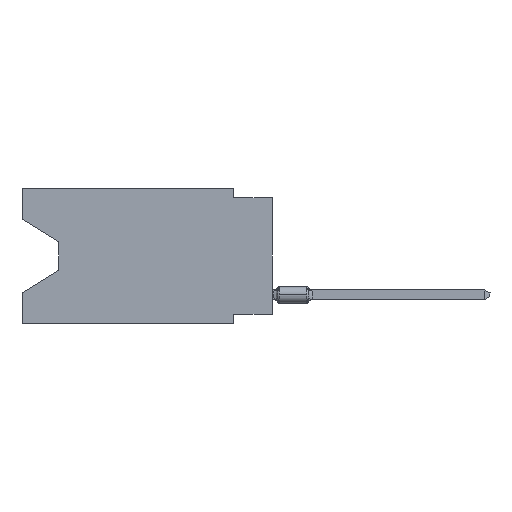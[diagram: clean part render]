
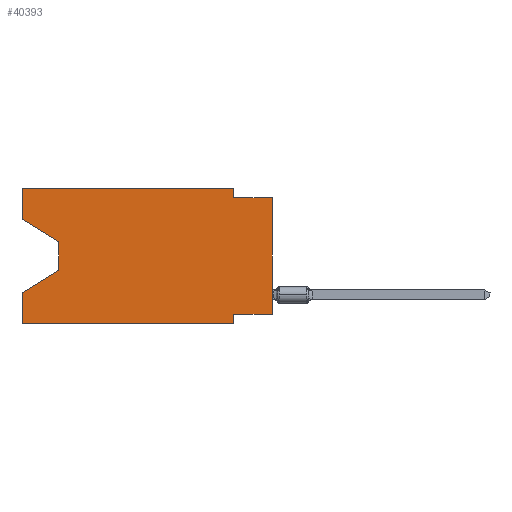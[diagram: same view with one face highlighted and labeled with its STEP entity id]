
A CAD part, left-side view. The second image highlights one B-rep face of the part: STEP entity #40393.
In plain terms, the highlighted planar face has unit normal (-1, 0, 0).
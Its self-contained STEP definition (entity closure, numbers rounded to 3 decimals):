
#534 = CARTESIAN_POINT ( 'NONE',  ( 0., 16.383, 0. ) ) ;
#1116 = CARTESIAN_POINT ( 'NONE',  ( 0., 16.383, 0. ) ) ;
#1159 = LINE ( 'NONE', #534, #43737 ) ;
#1379 = LINE ( 'NONE', #24258, #45054 ) ;
#1536 = DIRECTION ( 'NONE',  ( 0., 0., -1. ) ) ;
#2438 = EDGE_LOOP ( 'NONE', ( #58298, #54581, #25618, #20594, #7840, #58478, #11029, #13163, #11978, #22120, #38118, #57134 ) ) ;
#2689 = EDGE_CURVE ( 'NONE', #57153, #38139, #52926, .T. ) ;
#3599 = EDGE_CURVE ( 'NONE', #52192, #25789, #53669, .T. ) ;
#4442 = VECTOR ( 'NONE', #15728, 1000. ) ;
#5353 = DIRECTION ( 'NONE',  ( 0., 0., -1. ) ) ;
#6233 = FACE_OUTER_BOUND ( 'NONE', #2438, .T. ) ;
#7737 = EDGE_CURVE ( 'NONE', #38989, #37722, #52046, .T. ) ;
#7840 = ORIENTED_EDGE ( 'NONE', *, *, #38805, .T. ) ;
#7845 = CARTESIAN_POINT ( 'NONE',  ( 0., 13.97, -5.385 ) ) ;
#9365 = DIRECTION ( 'NONE',  ( 0., 0., 1. ) ) ;
#10062 = VERTEX_POINT ( 'NONE', #35258 ) ;
#10211 = CARTESIAN_POINT ( 'NONE',  ( 0., 16.383, 0. ) ) ;
#11029 = ORIENTED_EDGE ( 'NONE', *, *, #59917, .F. ) ;
#11051 = EDGE_CURVE ( 'NONE', #14133, #39056, #57338, .T. ) ;
#11978 = ORIENTED_EDGE ( 'NONE', *, *, #13653, .F. ) ;
#12089 = LINE ( 'NONE', #25820, #41133 ) ;
#12208 = CARTESIAN_POINT ( 'NONE',  ( 0., 16.383, -8.89 ) ) ;
#13156 = EDGE_CURVE ( 'NONE', #53012, #34912, #12089, .T. ) ;
#13163 = ORIENTED_EDGE ( 'NONE', *, *, #3599, .T. ) ;
#13304 = EDGE_CURVE ( 'NONE', #10062, #37722, #45962, .T. ) ;
#13653 = EDGE_CURVE ( 'NONE', #48090, #25789, #21405, .T. ) ;
#13807 = EDGE_CURVE ( 'NONE', #38139, #48090, #1379, .T. ) ;
#14133 = VERTEX_POINT ( 'NONE', #50762 ) ;
#15728 = DIRECTION ( 'NONE',  ( 0., -1., 0. ) ) ;
#16713 = VECTOR ( 'NONE', #56266, 1000. ) ;
#17088 = LINE ( 'NONE', #12208, #52303 ) ;
#19341 = CARTESIAN_POINT ( 'NONE',  ( 0., 2.54, -0.635 ) ) ;
#19373 = CARTESIAN_POINT ( 'NONE',  ( 0., 16.383, -2.038 ) ) ;
#20360 = DIRECTION ( 'NONE',  ( 0., -0.855, -0.519 ) ) ;
#20594 = ORIENTED_EDGE ( 'NONE', *, *, #7737, .F. ) ;
#21405 = LINE ( 'NONE', #31171, #56774 ) ;
#21551 = DIRECTION ( 'NONE',  ( 0., 0.855, -0.519 ) ) ;
#22120 = ORIENTED_EDGE ( 'NONE', *, *, #13807, .F. ) ;
#23295 = EDGE_CURVE ( 'NONE', #53012, #57153, #1159, .T. ) ;
#24258 = CARTESIAN_POINT ( 'NONE',  ( 0., 2.54, 0. ) ) ;
#24838 = PLANE ( 'NONE',  #38788 ) ;
#24875 = DIRECTION ( 'NONE',  ( 0., -1., 0. ) ) ;
#25618 = ORIENTED_EDGE ( 'NONE', *, *, #13304, .T. ) ;
#25625 = DIRECTION ( 'NONE',  ( 0., 0., 1. ) ) ;
#25789 = VERTEX_POINT ( 'NONE', #59652 ) ;
#25820 = CARTESIAN_POINT ( 'NONE',  ( 0., 16.383, -2.038 ) ) ;
#26841 = CARTESIAN_POINT ( 'NONE',  ( 0., 16.383, -6.852 ) ) ;
#26843 = VECTOR ( 'NONE', #51600, 1000. ) ;
#27988 = DIRECTION ( 'NONE',  ( 0., 0., 1. ) ) ;
#28391 = CARTESIAN_POINT ( 'NONE',  ( 0., 0., -8.255 ) ) ;
#31171 = CARTESIAN_POINT ( 'NONE',  ( 0., 0., -0.635 ) ) ;
#34187 = EDGE_CURVE ( 'NONE', #34912, #10062, #51899, .T. ) ;
#34273 = DIRECTION ( 'NONE',  ( 1., 0., 0. ) ) ;
#34309 = CARTESIAN_POINT ( 'NONE',  ( 0., 16.383, 0. ) ) ;
#34912 = VERTEX_POINT ( 'NONE', #37631 ) ;
#35258 = CARTESIAN_POINT ( 'NONE',  ( 0., 13.97, -5.385 ) ) ;
#37631 = CARTESIAN_POINT ( 'NONE',  ( 0., 13.97, -3.505 ) ) ;
#37722 = VERTEX_POINT ( 'NONE', #26841 ) ;
#37968 = VECTOR ( 'NONE', #9365, 1000. ) ;
#38118 = ORIENTED_EDGE ( 'NONE', *, *, #2689, .F. ) ;
#38139 = VERTEX_POINT ( 'NONE', #45071 ) ;
#38788 = AXIS2_PLACEMENT_3D ( 'NONE', #47718, #34273, #48309 ) ;
#38805 = EDGE_CURVE ( 'NONE', #38989, #39056, #17088, .T. ) ;
#38989 = VERTEX_POINT ( 'NONE', #40880 ) ;
#39056 = VERTEX_POINT ( 'NONE', #56095 ) ;
#39057 = CARTESIAN_POINT ( 'NONE',  ( 0., 0., 0. ) ) ;
#40393 = ADVANCED_FACE ( 'NONE', ( #6233 ), #24838, .F. ) ;
#40880 = CARTESIAN_POINT ( 'NONE',  ( 0., 16.383, -8.89 ) ) ;
#41133 = VECTOR ( 'NONE', #20360, 1000. ) ;
#42539 = CARTESIAN_POINT ( 'NONE',  ( 0., 0., -8.255 ) ) ;
#43737 = VECTOR ( 'NONE', #27988, 1000. ) ;
#45054 = VECTOR ( 'NONE', #5353, 1000. ) ;
#45071 = CARTESIAN_POINT ( 'NONE',  ( 0., 2.54, 0. ) ) ;
#45962 = LINE ( 'NONE', #7845, #47948 ) ;
#47718 = CARTESIAN_POINT ( 'NONE',  ( 0., 16.383, 0. ) ) ;
#47948 = VECTOR ( 'NONE', #21551, 1000. ) ;
#48090 = VERTEX_POINT ( 'NONE', #19341 ) ;
#48309 = DIRECTION ( 'NONE',  ( 0., 0., -1. ) ) ;
#48484 = CARTESIAN_POINT ( 'NONE',  ( 0., 2.54, -8.89 ) ) ;
#49185 = VECTOR ( 'NONE', #25625, 1000. ) ;
#50762 = CARTESIAN_POINT ( 'NONE',  ( 0., 2.54, -8.255 ) ) ;
#51600 = DIRECTION ( 'NONE',  ( 0., 0., -1. ) ) ;
#51826 = VECTOR ( 'NONE', #1536, 1000. ) ;
#51899 = LINE ( 'NONE', #53594, #26843 ) ;
#52046 = LINE ( 'NONE', #1116, #37968 ) ;
#52192 = VERTEX_POINT ( 'NONE', #28391 ) ;
#52303 = VECTOR ( 'NONE', #58861, 1000. ) ;
#52926 = LINE ( 'NONE', #34309, #4442 ) ;
#53012 = VERTEX_POINT ( 'NONE', #19373 ) ;
#53594 = CARTESIAN_POINT ( 'NONE',  ( 0., 13.97, -3.505 ) ) ;
#53669 = LINE ( 'NONE', #39057, #49185 ) ;
#54581 = ORIENTED_EDGE ( 'NONE', *, *, #34187, .T. ) ;
#56095 = CARTESIAN_POINT ( 'NONE',  ( 0., 2.54, -8.89 ) ) ;
#56266 = DIRECTION ( 'NONE',  ( 0., 1., 0. ) ) ;
#56774 = VECTOR ( 'NONE', #24875, 1000. ) ;
#57134 = ORIENTED_EDGE ( 'NONE', *, *, #23295, .F. ) ;
#57153 = VERTEX_POINT ( 'NONE', #10211 ) ;
#57338 = LINE ( 'NONE', #48484, #51826 ) ;
#58298 = ORIENTED_EDGE ( 'NONE', *, *, #13156, .T. ) ;
#58478 = ORIENTED_EDGE ( 'NONE', *, *, #11051, .F. ) ;
#58861 = DIRECTION ( 'NONE',  ( 0., -1., 0. ) ) ;
#59652 = CARTESIAN_POINT ( 'NONE',  ( 0., 0., -0.635 ) ) ;
#59917 = EDGE_CURVE ( 'NONE', #52192, #14133, #60244, .T. ) ;
#60244 = LINE ( 'NONE', #42539, #16713 ) ;
